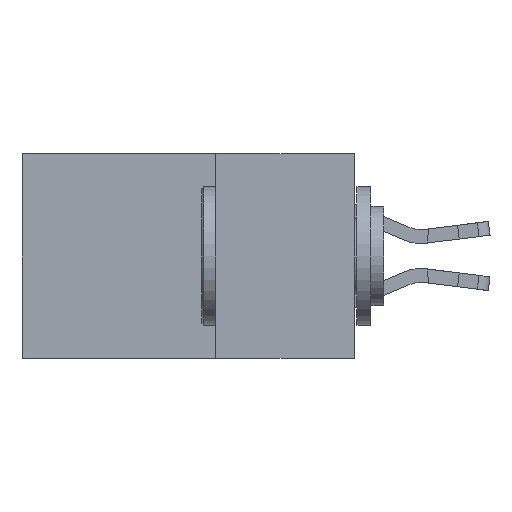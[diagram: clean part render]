
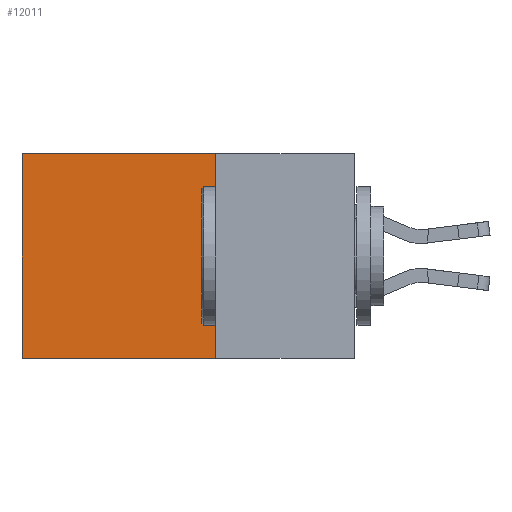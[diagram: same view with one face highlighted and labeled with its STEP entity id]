
A CAD part, left-side view. The second image highlights one B-rep face of the part: STEP entity #12011.
In plain terms, the highlighted planar face has unit normal (-1, 0, 0).
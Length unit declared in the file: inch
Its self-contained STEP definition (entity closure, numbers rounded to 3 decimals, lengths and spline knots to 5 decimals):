
#625 = ORIENTED_EDGE ( 'NONE', *, *, #5758, .F. ) ;
#1149 = ORIENTED_EDGE ( 'NONE', *, *, #11246, .T. ) ;
#1189 = PLANE ( 'NONE',  #15902 ) ;
#1396 = LINE ( 'NONE', #16853, #4638 ) ;
#1585 = LINE ( 'NONE', #1781, #14421 ) ;
#1781 = CARTESIAN_POINT ( 'NONE',  ( 0.2615, 0.25, 0. ) ) ;
#2136 = VERTEX_POINT ( 'NONE', #18078 ) ;
#2661 = FACE_OUTER_BOUND ( 'NONE', #10575, .T. ) ;
#3047 = VECTOR ( 'NONE', #6409, 39.37008 ) ;
#3937 = DIRECTION ( 'NONE',  ( 1., 0., 0. ) ) ;
#4200 = VERTEX_POINT ( 'NONE', #13529 ) ;
#4565 = ORIENTED_EDGE ( 'NONE', *, *, #13043, .F. ) ;
#4638 = VECTOR ( 'NONE', #10938, 39.37008 ) ;
#4752 = VERTEX_POINT ( 'NONE', #16973 ) ;
#5758 = EDGE_CURVE ( 'NONE', #2136, #4200, #17711, .T. ) ;
#6063 = ORIENTED_EDGE ( 'NONE', *, *, #9159, .T. ) ;
#6409 = DIRECTION ( 'NONE',  ( 0., 1., 0. ) ) ;
#8295 = DIRECTION ( 'NONE',  ( 0., 0., -1. ) ) ;
#8515 = CARTESIAN_POINT ( 'NONE',  ( 0.2615, 0.25, 0. ) ) ;
#8668 = LINE ( 'NONE', #17281, #13577 ) ;
#9159 = EDGE_CURVE ( 'NONE', #4752, #4200, #1396, .T. ) ;
#9891 = DIRECTION ( 'NONE',  ( 0., 0., -1. ) ) ;
#10575 = EDGE_LOOP ( 'NONE', ( #6063, #625, #4565, #1149 ) ) ;
#10681 = CARTESIAN_POINT ( 'NONE',  ( 0.2615, 0.25, -0.37 ) ) ;
#10938 = DIRECTION ( 'NONE',  ( 0., 0., -1. ) ) ;
#11246 = EDGE_CURVE ( 'NONE', #14295, #4752, #1585, .T. ) ;
#12011 = ADVANCED_FACE ( 'NONE', ( #2661 ), #1189, .F. ) ;
#13043 = EDGE_CURVE ( 'NONE', #14295, #2136, #8668, .T. ) ;
#13058 = DIRECTION ( 'NONE',  ( 0., 1., 0. ) ) ;
#13529 = CARTESIAN_POINT ( 'NONE',  ( 0.2615, 0.6, -0.37 ) ) ;
#13577 = VECTOR ( 'NONE', #9891, 39.37008 ) ;
#14295 = VERTEX_POINT ( 'NONE', #8515 ) ;
#14421 = VECTOR ( 'NONE', #13058, 39.37008 ) ;
#15902 = AXIS2_PLACEMENT_3D ( 'NONE', #16448, #3937, #8295 ) ;
#16448 = CARTESIAN_POINT ( 'NONE',  ( 0.2615, 0.25, -0.37 ) ) ;
#16853 = CARTESIAN_POINT ( 'NONE',  ( 0.2615, 0.6, -0.37 ) ) ;
#16973 = CARTESIAN_POINT ( 'NONE',  ( 0.2615, 0.6, 0. ) ) ;
#17281 = CARTESIAN_POINT ( 'NONE',  ( 0.2615, 0.25, -0.37 ) ) ;
#17711 = LINE ( 'NONE', #10681, #3047 ) ;
#18078 = CARTESIAN_POINT ( 'NONE',  ( 0.2615, 0.25, -0.37 ) ) ;
